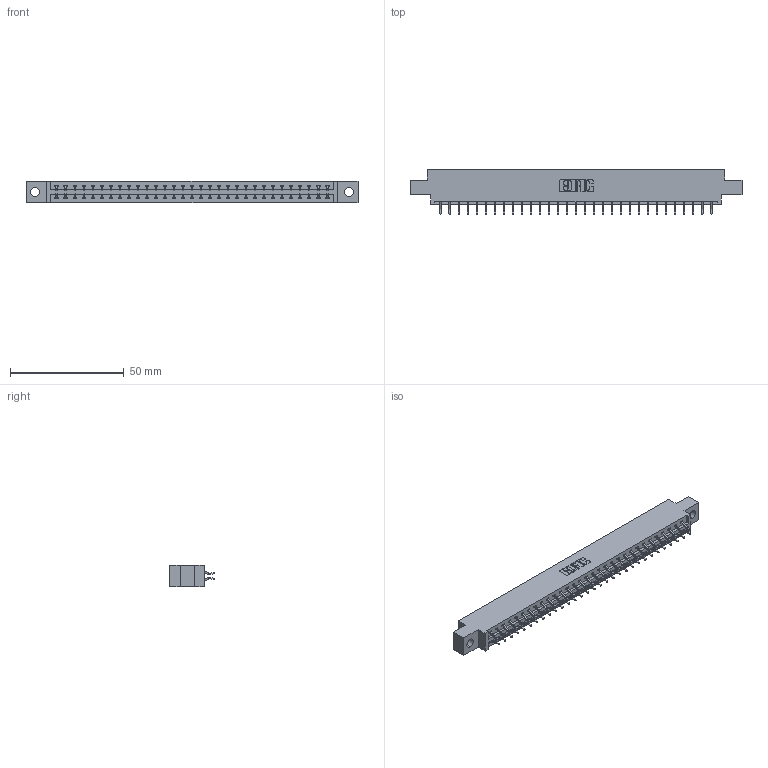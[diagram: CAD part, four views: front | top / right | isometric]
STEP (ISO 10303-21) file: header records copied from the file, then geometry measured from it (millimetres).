
FILE_DESCRIPTION (( 'STEP AP203' ), '1' );
FILE_NAME ('337-062-556-804.STEP', '2018-08-11T04:44:57', ( '' ), ( '' ), 'SwSTEP 2.0', 'SolidWorks 2016', '' );
FILE_SCHEMA (( 'CONFIG_CONTROL_DESIGN' ));
Length unit declared in the file: inch
Products named in the file (3): 337 Part_0.170 Offset - 0.156 Dia-TH; 345-292-001_556 Tail; 337-062-556-804
Assembly tree (63 placements, depth 2):
  337-062-556-804
    337 Part_0.170 Offset - 0.156 Dia-TH
    345-292-001_556 Tail  x62
Bounding box: 145.85 x 19.57 x 9.4 mm (x, y, z)
Volume: 15016.3 mm3; surface area: 16708.9 mm2
Topology: 63 solids, 63 shells, 3838 faces, 11421 edges, 7530 vertices
Faces by surface type: plane 2678, cylinder 1160
Entity records: 25813 total; most frequent: CARTESIAN_POINT 4374, ORIENTED_EDGE 4298, DIRECTION 3729, EDGE_CURVE 2149, VECTOR 2013, LINE 2013, VERTEX_POINT 1430, AXIS2_PLACEMENT_3D 858
